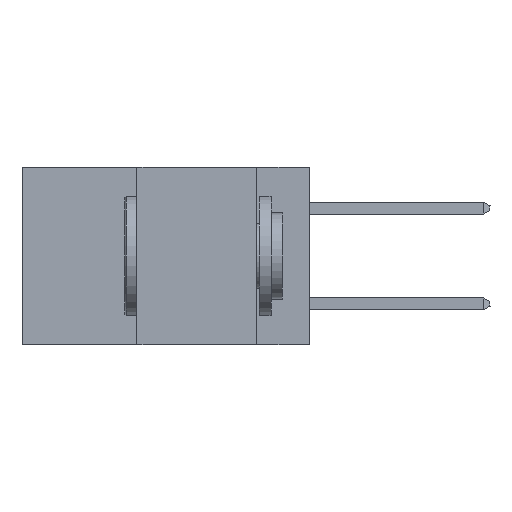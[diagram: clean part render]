
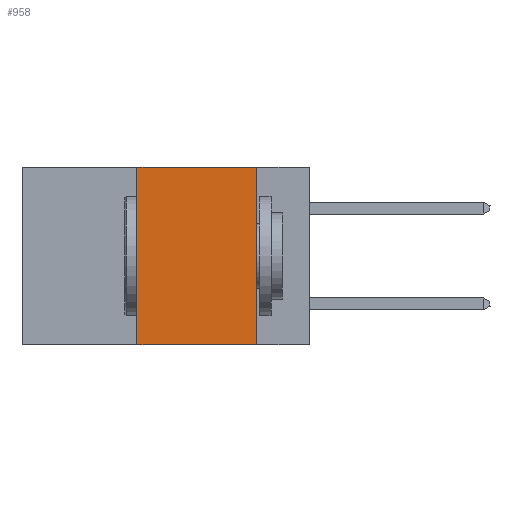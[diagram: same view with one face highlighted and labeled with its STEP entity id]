
A CAD part, left-side view. The second image highlights one B-rep face of the part: STEP entity #958.
In plain terms, the highlighted planar face has unit normal (-1, 0, 0).
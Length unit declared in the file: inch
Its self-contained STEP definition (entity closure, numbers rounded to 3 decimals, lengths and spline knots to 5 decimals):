
#568 = CARTESIAN_POINT ( 'NONE',  ( 0., 0.36, 0. ) ) ;
#849 = VERTEX_POINT ( 'NONE', #15263 ) ;
#958 = ADVANCED_FACE ( 'NONE', ( #12416 ), #7182, .F. ) ;
#3282 = VECTOR ( 'NONE', #26508, 39.37008 ) ;
#4021 = LINE ( 'NONE', #26499, #15346 ) ;
#4888 = DIRECTION ( 'NONE',  ( 0., -1., 0. ) ) ;
#4898 = CARTESIAN_POINT ( 'NONE',  ( 0., 0.36, 0. ) ) ;
#6876 = DIRECTION ( 'NONE',  ( 0., 0., -1. ) ) ;
#6975 = DIRECTION ( 'NONE',  ( 1., 0., 0. ) ) ;
#7182 = PLANE ( 'NONE',  #25381 ) ;
#7217 = CARTESIAN_POINT ( 'NONE',  ( 0., 0.6, 0. ) ) ;
#7610 = VERTEX_POINT ( 'NONE', #568 ) ;
#8240 = VECTOR ( 'NONE', #12439, 39.37008 ) ;
#9263 = ORIENTED_EDGE ( 'NONE', *, *, #17687, .F. ) ;
#10837 = CARTESIAN_POINT ( 'NONE',  ( 0., 0.36, -0.37 ) ) ;
#10961 = LINE ( 'NONE', #24526, #29232 ) ;
#11119 = VERTEX_POINT ( 'NONE', #10837 ) ;
#11527 = ORIENTED_EDGE ( 'NONE', *, *, #18922, .T. ) ;
#12416 = FACE_OUTER_BOUND ( 'NONE', #31157, .T. ) ;
#12439 = DIRECTION ( 'NONE',  ( 0., -1., 0. ) ) ;
#13871 = LINE ( 'NONE', #26750, #8240 ) ;
#15000 = DIRECTION ( 'NONE',  ( 0., 0., -1. ) ) ;
#15263 = CARTESIAN_POINT ( 'NONE',  ( 0., 0.11, -0.37 ) ) ;
#15346 = VECTOR ( 'NONE', #4888, 39.37008 ) ;
#16832 = CARTESIAN_POINT ( 'NONE',  ( 0., 0.11, 0. ) ) ;
#17687 = EDGE_CURVE ( 'NONE', #18162, #849, #10961, .T. ) ;
#18162 = VERTEX_POINT ( 'NONE', #16832 ) ;
#18922 = EDGE_CURVE ( 'NONE', #11119, #849, #13871, .T. ) ;
#19571 = EDGE_CURVE ( 'NONE', #7610, #18162, #4021, .T. ) ;
#21984 = ORIENTED_EDGE ( 'NONE', *, *, #19571, .F. ) ;
#23493 = ORIENTED_EDGE ( 'NONE', *, *, #27901, .F. ) ;
#24526 = CARTESIAN_POINT ( 'NONE',  ( 0., 0.11, 0. ) ) ;
#25381 = AXIS2_PLACEMENT_3D ( 'NONE', #7217, #6975, #6876 ) ;
#26499 = CARTESIAN_POINT ( 'NONE',  ( 0., 0.6, 0. ) ) ;
#26508 = DIRECTION ( 'NONE',  ( 0., 0., 1. ) ) ;
#26750 = CARTESIAN_POINT ( 'NONE',  ( 0., 0.6, -0.37 ) ) ;
#27901 = EDGE_CURVE ( 'NONE', #11119, #7610, #28845, .T. ) ;
#28845 = LINE ( 'NONE', #4898, #3282 ) ;
#29232 = VECTOR ( 'NONE', #15000, 39.37008 ) ;
#31157 = EDGE_LOOP ( 'NONE', ( #9263, #21984, #23493, #11527 ) ) ;
